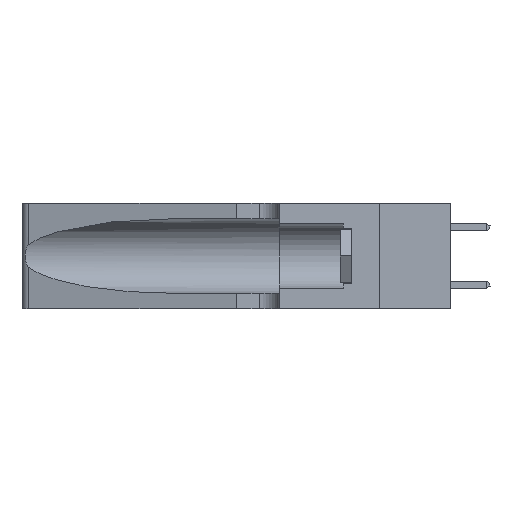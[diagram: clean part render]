
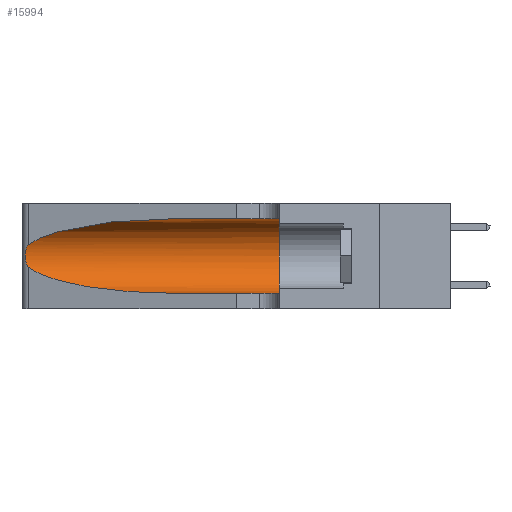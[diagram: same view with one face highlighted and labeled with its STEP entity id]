
A CAD part, left-side view. The second image highlights one B-rep face of the part: STEP entity #15994.
In plain terms, the highlighted cylindrical face has radius 3.308 mm (diameter 6.617 mm), a partial arc.
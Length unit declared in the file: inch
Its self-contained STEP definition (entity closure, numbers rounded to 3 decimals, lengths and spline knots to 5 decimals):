
#332 = EDGE_CURVE ( 'NONE', #4016, #28280, #36325, .T. ) ;
#1085 = CARTESIAN_POINT ( 'NONE',  ( 0.2373, 1.15595, 0.08982 ) ) ;
#2216 = CARTESIAN_POINT ( 'NONE',  ( 0.25639, 1.23186, 0.15144 ) ) ;
#3169 = LINE ( 'NONE', #38549, #34030 ) ;
#3411 = AXIS2_PLACEMENT_3D ( 'NONE', #48049, #22293, #3452 ) ;
#3452 = DIRECTION ( 'NONE',  ( 0., 0., -1. ) ) ;
#3461 = CYLINDRICAL_SURFACE ( 'NONE', #3411, 0.13025 ) ;
#3726 = VERTEX_POINT ( 'NONE', #32254 ) ;
#4016 = VERTEX_POINT ( 'NONE', #12834 ) ;
#4355 = EDGE_CURVE ( 'NONE', #3726, #41412, #3169, .T. ) ;
#5592 = ORIENTED_EDGE ( 'NONE', *, *, #16823, .F. ) ;
#5785 = CARTESIAN_POINT ( 'NONE',  ( 0.25787, 1.23484, 0.2124 ) ) ;
#5944 = CARTESIAN_POINT ( 'NONE',  ( 0.25487, 1.22718, 0.14631 ) ) ;
#6266 = CARTESIAN_POINT ( 'NONE',  ( 0.26075, 1.23896, 0.19203 ) ) ;
#6737 = DIRECTION ( 'NONE',  ( 0., -1., 0. ) ) ;
#7390 = EDGE_LOOP ( 'NONE', ( #25472, #10425, #46124, #21752, #5592, #40545 ) ) ;
#7638 = CARTESIAN_POINT ( 'NONE',  ( 0.25487, 1.22718, 0.22369 ) ) ;
#7919 =( BOUNDED_CURVE ( )  B_SPLINE_CURVE ( 3, ( #42238, #1085, #30827, #9501 ),
 .UNSPECIFIED., .F., .F. ) 
 B_SPLINE_CURVE_WITH_KNOTS ( ( 4, 4 ),
 ( 3.44316, 4.71239 ),
 .UNSPECIFIED. ) 
 CURVE ( )  GEOMETRIC_REPRESENTATION_ITEM ( )  RATIONAL_B_SPLINE_CURVE ( ( 1., 0.87, 0.87, 1. ) ) 
 REPRESENTATION_ITEM ( '' )  );
#9501 = CARTESIAN_POINT ( 'NONE',  ( 0.1305, 0.72297, 0.05475 ) ) ;
#9507 = CARTESIAN_POINT ( 'NONE',  ( 0.26018, 1.23835, 0.19895 ) ) ;
#9836 = CARTESIAN_POINT ( 'NONE',  ( 0.25639, 1.23184, 0.21858 ) ) ;
#10035 = CARTESIAN_POINT ( 'NONE',  ( 0.1305, 0.35, 0.05475 ) ) ;
#10425 = ORIENTED_EDGE ( 'NONE', *, *, #17652, .T. ) ;
#11018 = FACE_OUTER_BOUND ( 'NONE', #7390, .T. ) ;
#12834 = CARTESIAN_POINT ( 'NONE',  ( 0.1305, 0.72297, 0.31525 ) ) ;
#13268 = CARTESIAN_POINT ( 'NONE',  ( 0.26075, 1.23896, 0.178 ) ) ;
#14477 =( BOUNDED_CURVE ( )  B_SPLINE_CURVE ( 3, ( #40621, #29221, #44044, #21868 ),
 .UNSPECIFIED., .F., .T. ) 
 B_SPLINE_CURVE_WITH_KNOTS ( ( 4, 4 ),
 ( 1.5708, 2.84003 ),
 .UNSPECIFIED. ) 
 CURVE ( )  GEOMETRIC_REPRESENTATION_ITEM ( )  RATIONAL_B_SPLINE_CURVE ( ( 1., 0.87, 0.87, 1. ) ) 
 REPRESENTATION_ITEM ( '' )  );
#15615 = EDGE_CURVE ( 'NONE', #36639, #3726, #7919, .T. ) ;
#15994 = ADVANCED_FACE ( 'NONE', ( #11018 ), #3461, .F. ) ;
#16823 = EDGE_CURVE ( 'NONE', #28280, #41412, #39346, .T. ) ;
#17652 = EDGE_CURVE ( 'NONE', #36699, #36639, #23100, .T. ) ;
#19293 = CARTESIAN_POINT ( 'NONE',  ( 0.1305, 0.35, 0.185 ) ) ;
#19343 = EDGE_CURVE ( 'NONE', #4016, #36699, #14477, .T. ) ;
#20737 = CARTESIAN_POINT ( 'NONE',  ( 0.26017, 1.23833, 0.17102 ) ) ;
#21752 = ORIENTED_EDGE ( 'NONE', *, *, #4355, .T. ) ;
#21868 = CARTESIAN_POINT ( 'NONE',  ( 0.25487, 1.22718, 0.22369 ) ) ;
#22293 = DIRECTION ( 'NONE',  ( 0., -1., 0. ) ) ;
#23049 = DIRECTION ( 'NONE',  ( 0., 0., 1. ) ) ;
#23100 = B_SPLINE_CURVE_WITH_KNOTS ( 'NONE', 3,
 ( #46623, #28402, #9836, #5785, #28553, #9507, #6266, #13268, #20737, #35897, #24471, #2216, #28243, #5944 ),
 .UNSPECIFIED., .F., .F.,
 ( 4, 2, 2, 2, 2, 2, 4 ),
 ( 0., 0.00027, 0.00053, 0.00107, 0.0016, 0.00187, 0.00214 ),
 .UNSPECIFIED. ) ;
#24471 = CARTESIAN_POINT ( 'NONE',  ( 0.25789, 1.23486, 0.15765 ) ) ;
#24936 = CARTESIAN_POINT ( 'NONE',  ( 0.1305, 1.61858, 0.31525 ) ) ;
#25472 = ORIENTED_EDGE ( 'NONE', *, *, #19343, .T. ) ;
#27788 = DIRECTION ( 'NONE',  ( 0., -1., 0. ) ) ;
#28243 = CARTESIAN_POINT ( 'NONE',  ( 0.25555, 1.22993, 0.14849 ) ) ;
#28280 = VERTEX_POINT ( 'NONE', #45223 ) ;
#28402 = CARTESIAN_POINT ( 'NONE',  ( 0.25555, 1.22994, 0.2215 ) ) ;
#28553 = CARTESIAN_POINT ( 'NONE',  ( 0.25854, 1.2359, 0.20912 ) ) ;
#29221 = CARTESIAN_POINT ( 'NONE',  ( 0.18966, 0.96281, 0.31525 ) ) ;
#30073 = DIRECTION ( 'NONE',  ( 0., 1., 0. ) ) ;
#30081 = CARTESIAN_POINT ( 'NONE',  ( 0.25487, 1.22718, 0.14631 ) ) ;
#30827 = CARTESIAN_POINT ( 'NONE',  ( 0.18966, 0.96281, 0.05475 ) ) ;
#32254 = CARTESIAN_POINT ( 'NONE',  ( 0.1305, 0.72297, 0.05475 ) ) ;
#33976 = VECTOR ( 'NONE', #6737, 39.37008 ) ;
#34030 = VECTOR ( 'NONE', #27788, 39.37008 ) ;
#35897 = CARTESIAN_POINT ( 'NONE',  ( 0.25856, 1.23593, 0.16098 ) ) ;
#36325 = LINE ( 'NONE', #24936, #33976 ) ;
#36639 = VERTEX_POINT ( 'NONE', #30081 ) ;
#36699 = VERTEX_POINT ( 'NONE', #7638 ) ;
#38549 = CARTESIAN_POINT ( 'NONE',  ( 0.1305, 1.61858, 0.05475 ) ) ;
#39346 = CIRCLE ( 'NONE', #47407, 0.13025 ) ;
#40545 = ORIENTED_EDGE ( 'NONE', *, *, #332, .F. ) ;
#40621 = CARTESIAN_POINT ( 'NONE',  ( 0.1305, 0.72297, 0.31525 ) ) ;
#41412 = VERTEX_POINT ( 'NONE', #10035 ) ;
#42238 = CARTESIAN_POINT ( 'NONE',  ( 0.25487, 1.22718, 0.14631 ) ) ;
#44044 = CARTESIAN_POINT ( 'NONE',  ( 0.2373, 1.15595, 0.28018 ) ) ;
#45223 = CARTESIAN_POINT ( 'NONE',  ( 0.1305, 0.35, 0.31525 ) ) ;
#46124 = ORIENTED_EDGE ( 'NONE', *, *, #15615, .T. ) ;
#46623 = CARTESIAN_POINT ( 'NONE',  ( 0.25487, 1.22718, 0.22369 ) ) ;
#47407 = AXIS2_PLACEMENT_3D ( 'NONE', #19293, #30073, #23049 ) ;
#48049 = CARTESIAN_POINT ( 'NONE',  ( 0.1305, 1.61858, 0.185 ) ) ;
